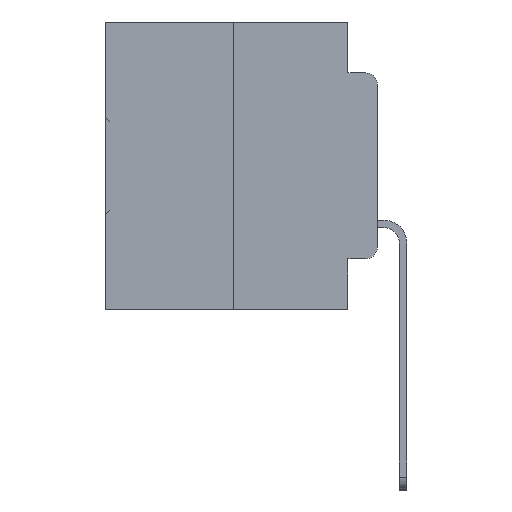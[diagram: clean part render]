
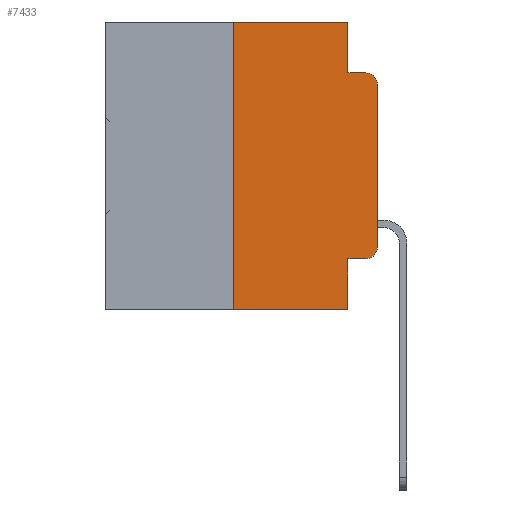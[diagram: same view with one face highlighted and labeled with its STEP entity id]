
A CAD part, left-side view. The second image highlights one B-rep face of the part: STEP entity #7433.
In plain terms, the highlighted planar face has unit normal (-1, 0, 0).
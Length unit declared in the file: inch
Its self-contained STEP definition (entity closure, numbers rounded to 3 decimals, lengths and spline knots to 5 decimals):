
#433 = LINE ( 'NONE', #32835, #1339 ) ;
#614 = ORIENTED_EDGE ( 'NONE', *, *, #17116, .F. ) ;
#1087 = DIRECTION ( 'NONE',  ( 0., 0., -1. ) ) ;
#1211 = CARTESIAN_POINT ( 'NONE',  ( 0., 0.25, -0.5 ) ) ;
#1339 = VECTOR ( 'NONE', #14891, 39.37008 ) ;
#2125 = DIRECTION ( 'NONE',  ( 1., 0., 0. ) ) ;
#2311 = DIRECTION ( 'NONE',  ( 0., -1., 0. ) ) ;
#2402 = LINE ( 'NONE', #16591, #16407 ) ;
#2665 = LINE ( 'NONE', #29466, #29471 ) ;
#2757 = ORIENTED_EDGE ( 'NONE', *, *, #18888, .F. ) ;
#3145 = CARTESIAN_POINT ( 'NONE',  ( 0., 0.051, -0.0885 ) ) ;
#3378 = DIRECTION ( 'NONE',  ( 0., -1., 0. ) ) ;
#4614 = FACE_OUTER_BOUND ( 'NONE', #23197, .T. ) ;
#4706 = CARTESIAN_POINT ( 'NONE',  ( 0., 0.051, -0.5 ) ) ;
#5852 = AXIS2_PLACEMENT_3D ( 'NONE', #17838, #2125, #20421 ) ;
#5935 = EDGE_CURVE ( 'NONE', #30956, #8909, #28674, .T. ) ;
#6180 = LINE ( 'NONE', #7302, #11544 ) ;
#6252 = DIRECTION ( 'NONE',  ( 0., -1., 0. ) ) ;
#6300 = VERTEX_POINT ( 'NONE', #28831 ) ;
#6668 = CARTESIAN_POINT ( 'NONE',  ( 0., 0.02, -0.1085 ) ) ;
#6716 = DIRECTION ( 'NONE',  ( 0., 0., 1. ) ) ;
#6766 = VERTEX_POINT ( 'NONE', #12586 ) ;
#7018 = DIRECTION ( 'NONE',  ( 0., 0., -1. ) ) ;
#7302 = CARTESIAN_POINT ( 'NONE',  ( 0., 0.051, 0. ) ) ;
#7433 = ADVANCED_FACE ( 'NONE', ( #4614 ), #15253, .F. ) ;
#8909 = VERTEX_POINT ( 'NONE', #12591 ) ;
#9273 = EDGE_CURVE ( 'NONE', #11281, #30962, #2665, .T. ) ;
#9342 = DIRECTION ( 'NONE',  ( 0., 0., -1. ) ) ;
#9475 = EDGE_CURVE ( 'NONE', #6766, #30956, #23017, .T. ) ;
#11176 = LINE ( 'NONE', #20604, #31707 ) ;
#11281 = VERTEX_POINT ( 'NONE', #1211 ) ;
#11440 = ORIENTED_EDGE ( 'NONE', *, *, #22264, .F. ) ;
#11544 = VECTOR ( 'NONE', #17794, 39.37008 ) ;
#11745 = VERTEX_POINT ( 'NONE', #18829 ) ;
#12586 = CARTESIAN_POINT ( 'NONE',  ( 0., 0., -0.3915 ) ) ;
#12591 = CARTESIAN_POINT ( 'NONE',  ( 0., 0.02, -0.0885 ) ) ;
#12635 = ORIENTED_EDGE ( 'NONE', *, *, #32577, .F. ) ;
#13887 = ORIENTED_EDGE ( 'NONE', *, *, #9273, .T. ) ;
#14467 = ORIENTED_EDGE ( 'NONE', *, *, #26343, .T. ) ;
#14652 = ORIENTED_EDGE ( 'NONE', *, *, #5935, .T. ) ;
#14691 = CARTESIAN_POINT ( 'NONE',  ( 0., 0.02, -0.4115 ) ) ;
#14839 = DIRECTION ( 'NONE',  ( 0., 0., 1. ) ) ;
#14891 = DIRECTION ( 'NONE',  ( 0., -1., 0. ) ) ;
#14985 = LINE ( 'NONE', #25154, #21825 ) ;
#15253 = PLANE ( 'NONE',  #5852 ) ;
#15263 = VERTEX_POINT ( 'NONE', #23851 ) ;
#16407 = VECTOR ( 'NONE', #3378, 39.37008 ) ;
#16591 = CARTESIAN_POINT ( 'NONE',  ( 0., 0.473, 0. ) ) ;
#16754 = VECTOR ( 'NONE', #6716, 39.37008 ) ;
#16880 = DIRECTION ( 'NONE',  ( -1., 0., 0. ) ) ;
#17116 = EDGE_CURVE ( 'NONE', #15263, #30962, #6180, .T. ) ;
#17538 = LINE ( 'NONE', #22292, #16754 ) ;
#17794 = DIRECTION ( 'NONE',  ( 0., 0., -1. ) ) ;
#17838 = CARTESIAN_POINT ( 'NONE',  ( 0., 0.473, 0. ) ) ;
#18829 = CARTESIAN_POINT ( 'NONE',  ( 0., 0.25, 0. ) ) ;
#18888 = EDGE_CURVE ( 'NONE', #11745, #6300, #2402, .T. ) ;
#20421 = DIRECTION ( 'NONE',  ( 0., 0., -1. ) ) ;
#20604 = CARTESIAN_POINT ( 'NONE',  ( 0., 0.051, -0.0885 ) ) ;
#21125 = ORIENTED_EDGE ( 'NONE', *, *, #25709, .F. ) ;
#21498 = CIRCLE ( 'NONE', #28615, 0.02 ) ;
#21825 = VECTOR ( 'NONE', #7018, 39.37008 ) ;
#22264 = EDGE_CURVE ( 'NONE', #11281, #11745, #17538, .T. ) ;
#22292 = CARTESIAN_POINT ( 'NONE',  ( 0., 0.25, 0. ) ) ;
#23017 = LINE ( 'NONE', #32784, #28247 ) ;
#23197 = EDGE_LOOP ( 'NONE', ( #31120, #14652, #12635, #21125, #2757, #11440, #13887, #614, #14467, #28158 ) ) ;
#23851 = CARTESIAN_POINT ( 'NONE',  ( 0., 0.051, -0.4115 ) ) ;
#24614 = EDGE_CURVE ( 'NONE', #24732, #6766, #21498, .T. ) ;
#24732 = VERTEX_POINT ( 'NONE', #14691 ) ;
#24813 = DIRECTION ( 'NONE',  ( -1., 0., 0. ) ) ;
#25154 = CARTESIAN_POINT ( 'NONE',  ( 0., 0.051, 0. ) ) ;
#25709 = EDGE_CURVE ( 'NONE', #6300, #29418, #14985, .T. ) ;
#26343 = EDGE_CURVE ( 'NONE', #15263, #24732, #433, .T. ) ;
#28158 = ORIENTED_EDGE ( 'NONE', *, *, #24614, .T. ) ;
#28247 = VECTOR ( 'NONE', #14839, 39.37008 ) ;
#28615 = AXIS2_PLACEMENT_3D ( 'NONE', #32223, #16880, #1087 ) ;
#28674 = CIRCLE ( 'NONE', #28815, 0.02 ) ;
#28815 = AXIS2_PLACEMENT_3D ( 'NONE', #6668, #24813, #9342 ) ;
#28831 = CARTESIAN_POINT ( 'NONE',  ( 0., 0.051, 0. ) ) ;
#29418 = VERTEX_POINT ( 'NONE', #3145 ) ;
#29466 = CARTESIAN_POINT ( 'NONE',  ( 0., 0.473, -0.5 ) ) ;
#29471 = VECTOR ( 'NONE', #6252, 39.37008 ) ;
#30552 = CARTESIAN_POINT ( 'NONE',  ( 0., 0., -0.1085 ) ) ;
#30956 = VERTEX_POINT ( 'NONE', #30552 ) ;
#30962 = VERTEX_POINT ( 'NONE', #4706 ) ;
#31120 = ORIENTED_EDGE ( 'NONE', *, *, #9475, .T. ) ;
#31707 = VECTOR ( 'NONE', #2311, 39.37008 ) ;
#32223 = CARTESIAN_POINT ( 'NONE',  ( 0., 0.02, -0.3915 ) ) ;
#32577 = EDGE_CURVE ( 'NONE', #29418, #8909, #11176, .T. ) ;
#32784 = CARTESIAN_POINT ( 'NONE',  ( 0., 0., 0. ) ) ;
#32835 = CARTESIAN_POINT ( 'NONE',  ( 0., 0.051, -0.4115 ) ) ;
